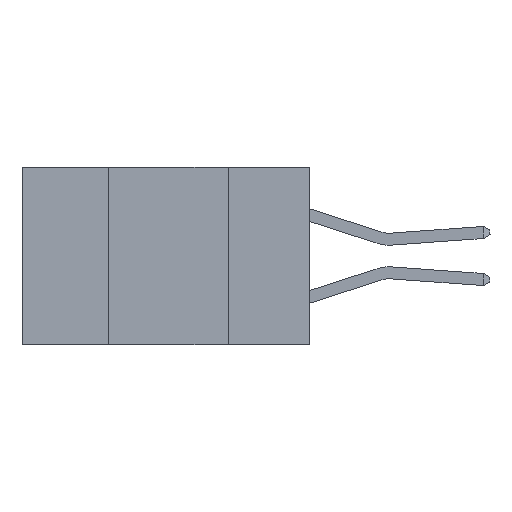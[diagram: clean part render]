
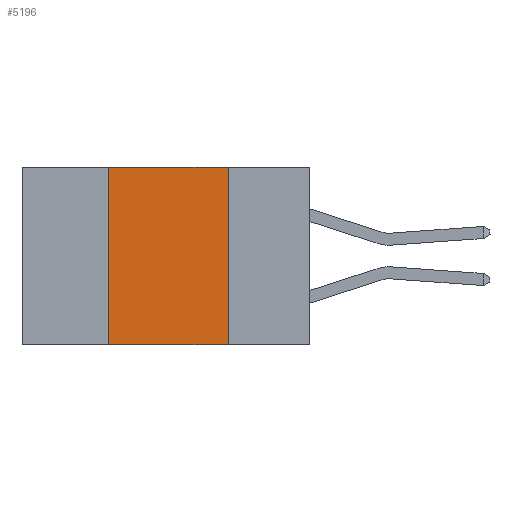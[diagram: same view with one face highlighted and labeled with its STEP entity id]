
A CAD part, left-side view. The second image highlights one B-rep face of the part: STEP entity #5196.
In plain terms, the highlighted planar face has unit normal (-1, 0, 0).
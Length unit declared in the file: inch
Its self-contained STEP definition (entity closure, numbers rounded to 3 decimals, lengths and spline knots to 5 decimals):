
#1302 = VERTEX_POINT ( 'NONE', #16152 ) ;
#1755 = LINE ( 'NONE', #25200, #6780 ) ;
#2888 = CARTESIAN_POINT ( 'NONE',  ( 0., 0.6, 0. ) ) ;
#3990 = CARTESIAN_POINT ( 'NONE',  ( 0., 0.42, 0. ) ) ;
#4424 = CARTESIAN_POINT ( 'NONE',  ( 0., 0.17, 0. ) ) ;
#5196 = ADVANCED_FACE ( 'NONE', ( #26485 ), #25462, .F. ) ;
#5313 = LINE ( 'NONE', #7479, #10243 ) ;
#6780 = VECTOR ( 'NONE', #15064, 39.37008 ) ;
#7145 = DIRECTION ( 'NONE',  ( 1., 0., 0. ) ) ;
#7479 = CARTESIAN_POINT ( 'NONE',  ( 0., 0.42, -0.37 ) ) ;
#8868 = CARTESIAN_POINT ( 'NONE',  ( 0., 0.17, -0.37 ) ) ;
#9515 = EDGE_CURVE ( 'NONE', #15371, #1302, #17425, .T. ) ;
#10243 = VECTOR ( 'NONE', #25951, 39.37008 ) ;
#12716 = VERTEX_POINT ( 'NONE', #23004 ) ;
#12810 = AXIS2_PLACEMENT_3D ( 'NONE', #2888, #7145, #21478 ) ;
#13641 = VECTOR ( 'NONE', #21204, 39.37008 ) ;
#14099 = EDGE_CURVE ( 'NONE', #12716, #1302, #14272, .T. ) ;
#14272 = LINE ( 'NONE', #25106, #13641 ) ;
#14482 = ORIENTED_EDGE ( 'NONE', *, *, #9515, .F. ) ;
#14602 = VERTEX_POINT ( 'NONE', #3990 ) ;
#14950 = ORIENTED_EDGE ( 'NONE', *, *, #14099, .T. ) ;
#15064 = DIRECTION ( 'NONE',  ( 0., -1., 0. ) ) ;
#15371 = VERTEX_POINT ( 'NONE', #4424 ) ;
#16152 = CARTESIAN_POINT ( 'NONE',  ( 0., 0.17, -0.37 ) ) ;
#16383 = EDGE_LOOP ( 'NONE', ( #14482, #23395, #24017, #14950 ) ) ;
#16800 = VECTOR ( 'NONE', #19016, 39.37008 ) ;
#17425 = LINE ( 'NONE', #8868, #16800 ) ;
#18184 = EDGE_CURVE ( 'NONE', #14602, #15371, #1755, .T. ) ;
#19016 = DIRECTION ( 'NONE',  ( 0., 0., -1. ) ) ;
#20952 = EDGE_CURVE ( 'NONE', #12716, #14602, #5313, .T. ) ;
#21204 = DIRECTION ( 'NONE',  ( 0., -1., 0. ) ) ;
#21478 = DIRECTION ( 'NONE',  ( 0., 0., -1. ) ) ;
#23004 = CARTESIAN_POINT ( 'NONE',  ( 0., 0.42, -0.37 ) ) ;
#23395 = ORIENTED_EDGE ( 'NONE', *, *, #18184, .F. ) ;
#24017 = ORIENTED_EDGE ( 'NONE', *, *, #20952, .F. ) ;
#25106 = CARTESIAN_POINT ( 'NONE',  ( 0., 0.6, -0.37 ) ) ;
#25200 = CARTESIAN_POINT ( 'NONE',  ( 0., 0.6, 0. ) ) ;
#25462 = PLANE ( 'NONE',  #12810 ) ;
#25951 = DIRECTION ( 'NONE',  ( 0., 0., 1. ) ) ;
#26485 = FACE_OUTER_BOUND ( 'NONE', #16383, .T. ) ;
